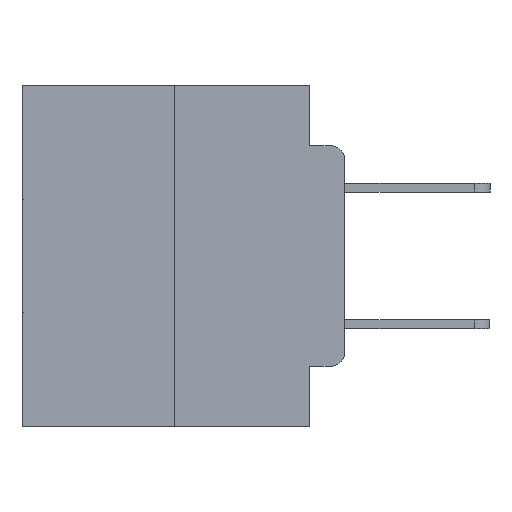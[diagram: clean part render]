
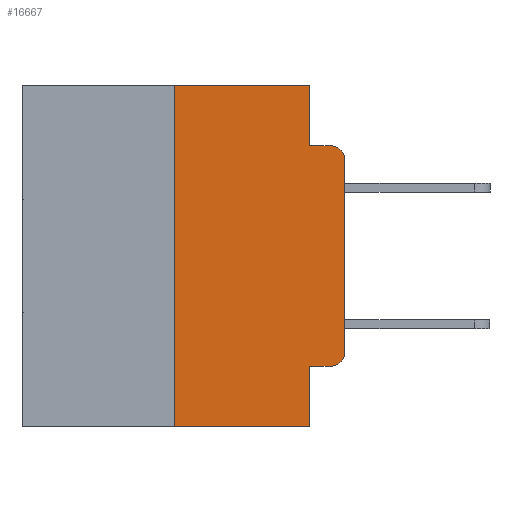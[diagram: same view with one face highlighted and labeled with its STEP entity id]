
A CAD part, left-side view. The second image highlights one B-rep face of the part: STEP entity #16667.
In plain terms, the highlighted planar face has unit normal (-1, 0, 0).
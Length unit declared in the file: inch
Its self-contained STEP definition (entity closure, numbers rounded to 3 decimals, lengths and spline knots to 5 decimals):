
#847 = LINE ( 'NONE', #28224, #5598 ) ;
#1088 = CARTESIAN_POINT ( 'NONE',  ( 0., 0.051, 0. ) ) ;
#1380 = PLANE ( 'NONE',  #16231 ) ;
#1430 = CIRCLE ( 'NONE', #13541, 0.02 ) ;
#1836 = CARTESIAN_POINT ( 'NONE',  ( 0., 0.02, -0.1085 ) ) ;
#1896 = DIRECTION ( 'NONE',  ( 0., -1., 0. ) ) ;
#1999 = DIRECTION ( 'NONE',  ( 0., 0., -1. ) ) ;
#2037 = VERTEX_POINT ( 'NONE', #3967 ) ;
#2121 = EDGE_CURVE ( 'NONE', #23424, #20337, #28192, .T. ) ;
#2884 = ORIENTED_EDGE ( 'NONE', *, *, #17419, .F. ) ;
#3151 = AXIS2_PLACEMENT_3D ( 'NONE', #1836, #17477, #4222 ) ;
#3233 = CARTESIAN_POINT ( 'NONE',  ( 0., 0.473, -0.5 ) ) ;
#3769 = DIRECTION ( 'NONE',  ( 0., 0., -1. ) ) ;
#3967 = CARTESIAN_POINT ( 'NONE',  ( 0., 0., -0.1085 ) ) ;
#4018 = EDGE_LOOP ( 'NONE', ( #11407, #20269, #18508, #2884, #14088, #18196, #9232, #19868, #21872, #25044 ) ) ;
#4222 = DIRECTION ( 'NONE',  ( 0., 0., -1. ) ) ;
#4765 = LINE ( 'NONE', #11154, #27200 ) ;
#5060 = VECTOR ( 'NONE', #13289, 39.37008 ) ;
#5598 = VECTOR ( 'NONE', #1999, 39.37008 ) ;
#6086 = VERTEX_POINT ( 'NONE', #6575 ) ;
#6575 = CARTESIAN_POINT ( 'NONE',  ( 0., 0.051, -0.4115 ) ) ;
#7124 = LINE ( 'NONE', #17528, #28151 ) ;
#7149 = LINE ( 'NONE', #13778, #11655 ) ;
#7172 = CARTESIAN_POINT ( 'NONE',  ( 0., 0.051, -0.5 ) ) ;
#8157 = VERTEX_POINT ( 'NONE', #13232 ) ;
#9002 = CARTESIAN_POINT ( 'NONE',  ( 0., 0.02, -0.4115 ) ) ;
#9178 = LINE ( 'NONE', #3233, #19490 ) ;
#9232 = ORIENTED_EDGE ( 'NONE', *, *, #23506, .T. ) ;
#9997 = EDGE_CURVE ( 'NONE', #19841, #8157, #1430, .T. ) ;
#10005 = CARTESIAN_POINT ( 'NONE',  ( 0., 0.02, -0.0885 ) ) ;
#10968 = CARTESIAN_POINT ( 'NONE',  ( 0., 0.02, -0.3915 ) ) ;
#10980 = VECTOR ( 'NONE', #28510, 39.37008 ) ;
#11102 = VERTEX_POINT ( 'NONE', #10005 ) ;
#11154 = CARTESIAN_POINT ( 'NONE',  ( 0., 0., 0. ) ) ;
#11407 = ORIENTED_EDGE ( 'NONE', *, *, #25987, .T. ) ;
#11521 = EDGE_CURVE ( 'NONE', #6086, #19841, #7149, .T. ) ;
#11655 = VECTOR ( 'NONE', #22471, 39.37008 ) ;
#11668 = LINE ( 'NONE', #15482, #5060 ) ;
#13199 = DIRECTION ( 'NONE',  ( 0., 0., -1. ) ) ;
#13232 = CARTESIAN_POINT ( 'NONE',  ( 0., 0., -0.3915 ) ) ;
#13289 = DIRECTION ( 'NONE',  ( 0., 0., -1. ) ) ;
#13541 = AXIS2_PLACEMENT_3D ( 'NONE', #10968, #26082, #13199 ) ;
#13778 = CARTESIAN_POINT ( 'NONE',  ( 0., 0.051, -0.4115 ) ) ;
#13829 = LINE ( 'NONE', #14777, #18945 ) ;
#13955 = CIRCLE ( 'NONE', #3151, 0.02 ) ;
#14088 = ORIENTED_EDGE ( 'NONE', *, *, #2121, .F. ) ;
#14298 = CARTESIAN_POINT ( 'NONE',  ( 0., 0.051, -0.0885 ) ) ;
#14451 = EDGE_CURVE ( 'NONE', #6086, #14633, #847, .T. ) ;
#14633 = VERTEX_POINT ( 'NONE', #7172 ) ;
#14777 = CARTESIAN_POINT ( 'NONE',  ( 0., 0.25, 0. ) ) ;
#14841 = CARTESIAN_POINT ( 'NONE',  ( 0., 0.473, 0. ) ) ;
#15324 = CARTESIAN_POINT ( 'NONE',  ( 0., 0.25, -0.5 ) ) ;
#15482 = CARTESIAN_POINT ( 'NONE',  ( 0., 0.051, 0. ) ) ;
#15942 = EDGE_CURVE ( 'NONE', #20601, #23424, #13829, .T. ) ;
#16231 = AXIS2_PLACEMENT_3D ( 'NONE', #14841, #17057, #3769 ) ;
#16667 = ADVANCED_FACE ( 'NONE', ( #24894 ), #1380, .F. ) ;
#17057 = DIRECTION ( 'NONE',  ( 1., 0., 0. ) ) ;
#17419 = EDGE_CURVE ( 'NONE', #20337, #22300, #11668, .T. ) ;
#17477 = DIRECTION ( 'NONE',  ( -1., 0., 0. ) ) ;
#17528 = CARTESIAN_POINT ( 'NONE',  ( 0., 0.051, -0.0885 ) ) ;
#18196 = ORIENTED_EDGE ( 'NONE', *, *, #15942, .F. ) ;
#18508 = ORIENTED_EDGE ( 'NONE', *, *, #23143, .F. ) ;
#18945 = VECTOR ( 'NONE', #27618, 39.37008 ) ;
#19490 = VECTOR ( 'NONE', #23012, 39.37008 ) ;
#19841 = VERTEX_POINT ( 'NONE', #9002 ) ;
#19868 = ORIENTED_EDGE ( 'NONE', *, *, #14451, .F. ) ;
#20269 = ORIENTED_EDGE ( 'NONE', *, *, #24548, .T. ) ;
#20337 = VERTEX_POINT ( 'NONE', #1088 ) ;
#20601 = VERTEX_POINT ( 'NONE', #15324 ) ;
#21872 = ORIENTED_EDGE ( 'NONE', *, *, #11521, .T. ) ;
#22086 = DIRECTION ( 'NONE',  ( 0., 0., 1. ) ) ;
#22300 = VERTEX_POINT ( 'NONE', #14298 ) ;
#22471 = DIRECTION ( 'NONE',  ( 0., -1., 0. ) ) ;
#23012 = DIRECTION ( 'NONE',  ( 0., -1., 0. ) ) ;
#23143 = EDGE_CURVE ( 'NONE', #22300, #11102, #7124, .T. ) ;
#23424 = VERTEX_POINT ( 'NONE', #26991 ) ;
#23506 = EDGE_CURVE ( 'NONE', #20601, #14633, #9178, .T. ) ;
#24548 = EDGE_CURVE ( 'NONE', #2037, #11102, #13955, .T. ) ;
#24894 = FACE_OUTER_BOUND ( 'NONE', #4018, .T. ) ;
#25044 = ORIENTED_EDGE ( 'NONE', *, *, #9997, .T. ) ;
#25987 = EDGE_CURVE ( 'NONE', #8157, #2037, #4765, .T. ) ;
#26082 = DIRECTION ( 'NONE',  ( -1., 0., 0. ) ) ;
#26991 = CARTESIAN_POINT ( 'NONE',  ( 0., 0.25, 0. ) ) ;
#27200 = VECTOR ( 'NONE', #22086, 39.37008 ) ;
#27618 = DIRECTION ( 'NONE',  ( 0., 0., 1. ) ) ;
#28151 = VECTOR ( 'NONE', #1896, 39.37008 ) ;
#28192 = LINE ( 'NONE', #28195, #10980 ) ;
#28195 = CARTESIAN_POINT ( 'NONE',  ( 0., 0.473, 0. ) ) ;
#28224 = CARTESIAN_POINT ( 'NONE',  ( 0., 0.051, 0. ) ) ;
#28510 = DIRECTION ( 'NONE',  ( 0., -1., 0. ) ) ;
